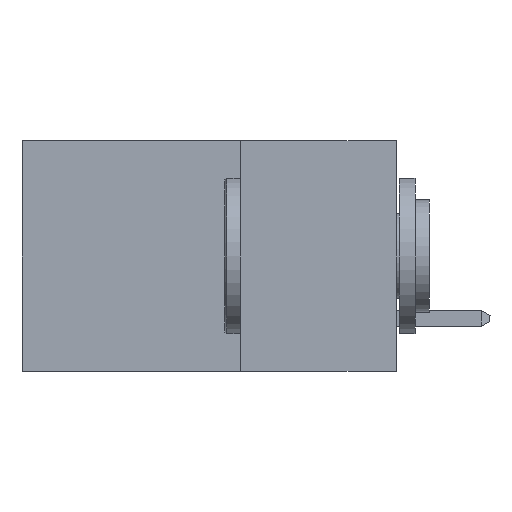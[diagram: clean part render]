
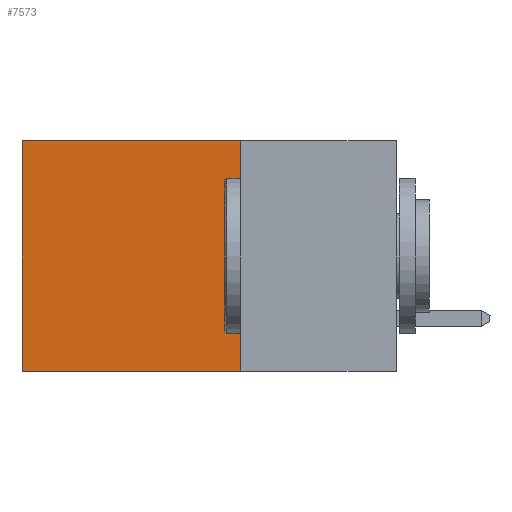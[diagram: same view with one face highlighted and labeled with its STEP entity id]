
A CAD part, left-side view. The second image highlights one B-rep face of the part: STEP entity #7573.
In plain terms, the highlighted planar face has unit normal (-1, 0, 0).
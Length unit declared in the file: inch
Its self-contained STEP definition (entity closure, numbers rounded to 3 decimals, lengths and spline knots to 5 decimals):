
#711 = EDGE_LOOP ( 'NONE', ( #2199, #4163, #9663, #10054 ) ) ;
#1696 = AXIS2_PLACEMENT_3D ( 'NONE', #9756, #9574, #9570 ) ;
#2199 = ORIENTED_EDGE ( 'NONE', *, *, #18044, .T. ) ;
#3838 = DIRECTION ( 'NONE',  ( 0., 0., -1. ) ) ;
#3946 = CARTESIAN_POINT ( 'NONE',  ( 0.2615, 0.25, -0.37 ) ) ;
#4163 = ORIENTED_EDGE ( 'NONE', *, *, #9870, .F. ) ;
#4518 = VERTEX_POINT ( 'NONE', #16304 ) ;
#4521 = CARTESIAN_POINT ( 'NONE',  ( 0.2615, 0.6, 0. ) ) ;
#7573 = ADVANCED_FACE ( 'NONE', ( #8460 ), #9675, .F. ) ;
#7876 = CARTESIAN_POINT ( 'NONE',  ( 0.2615, 0.6, -0.37 ) ) ;
#8074 = VERTEX_POINT ( 'NONE', #4521 ) ;
#8148 = EDGE_CURVE ( 'NONE', #4518, #13081, #17261, .T. ) ;
#8460 = FACE_OUTER_BOUND ( 'NONE', #711, .T. ) ;
#8648 = VECTOR ( 'NONE', #17804, 39.37008 ) ;
#9277 = CARTESIAN_POINT ( 'NONE',  ( 0.2615, 0.25, -0.37 ) ) ;
#9570 = DIRECTION ( 'NONE',  ( 0., 0., -1. ) ) ;
#9574 = DIRECTION ( 'NONE',  ( 1., 0., 0. ) ) ;
#9663 = ORIENTED_EDGE ( 'NONE', *, *, #8148, .F. ) ;
#9675 = PLANE ( 'NONE',  #1696 ) ;
#9756 = CARTESIAN_POINT ( 'NONE',  ( 0.2615, 0.25, -0.37 ) ) ;
#9870 = EDGE_CURVE ( 'NONE', #13081, #15340, #11014, .T. ) ;
#10054 = ORIENTED_EDGE ( 'NONE', *, *, #17216, .T. ) ;
#11014 = LINE ( 'NONE', #17761, #13695 ) ;
#12825 = VECTOR ( 'NONE', #3838, 39.37008 ) ;
#13081 = VERTEX_POINT ( 'NONE', #9277 ) ;
#13169 = VECTOR ( 'NONE', #14075, 39.37008 ) ;
#13695 = VECTOR ( 'NONE', #18399, 39.37008 ) ;
#14075 = DIRECTION ( 'NONE',  ( 0., 0., -1. ) ) ;
#14944 = CARTESIAN_POINT ( 'NONE',  ( 0.2615, 0.25, 0. ) ) ;
#15340 = VERTEX_POINT ( 'NONE', #18579 ) ;
#16304 = CARTESIAN_POINT ( 'NONE',  ( 0.2615, 0.25, 0. ) ) ;
#16796 = LINE ( 'NONE', #14944, #8648 ) ;
#17106 = LINE ( 'NONE', #7876, #13169 ) ;
#17216 = EDGE_CURVE ( 'NONE', #4518, #8074, #16796, .T. ) ;
#17261 = LINE ( 'NONE', #3946, #12825 ) ;
#17761 = CARTESIAN_POINT ( 'NONE',  ( 0.2615, 0.25, -0.37 ) ) ;
#17804 = DIRECTION ( 'NONE',  ( 0., 1., 0. ) ) ;
#18044 = EDGE_CURVE ( 'NONE', #8074, #15340, #17106, .T. ) ;
#18399 = DIRECTION ( 'NONE',  ( 0., 1., 0. ) ) ;
#18579 = CARTESIAN_POINT ( 'NONE',  ( 0.2615, 0.6, -0.37 ) ) ;
